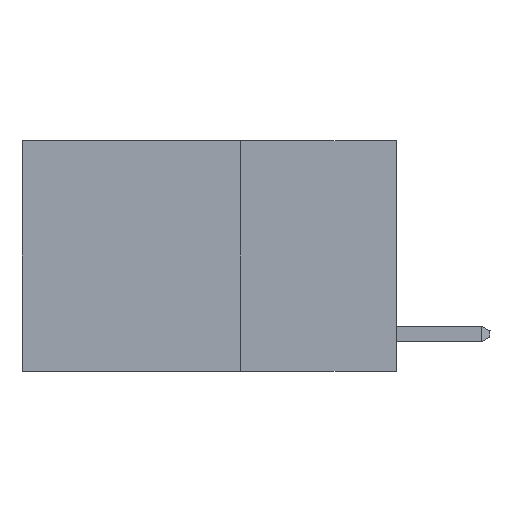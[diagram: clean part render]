
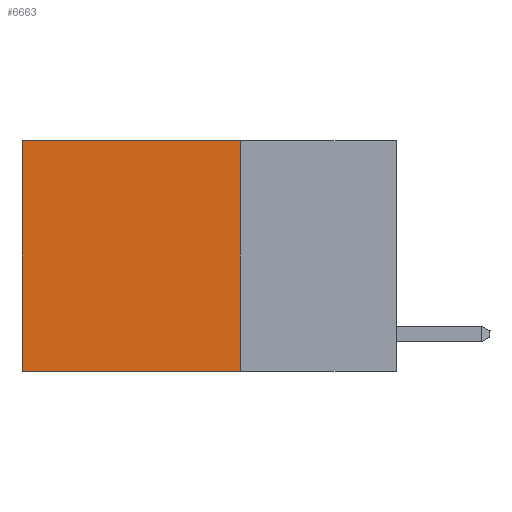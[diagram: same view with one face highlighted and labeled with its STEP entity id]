
A CAD part, left-side view. The second image highlights one B-rep face of the part: STEP entity #6663.
In plain terms, the highlighted planar face has unit normal (-1, 0, 0).
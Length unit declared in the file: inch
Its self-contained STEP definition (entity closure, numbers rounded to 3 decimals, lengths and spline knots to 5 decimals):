
#4 = CARTESIAN_POINT ( 'NONE',  ( 0.2625, 0.6, -0.37 ) ) ;
#720 = VECTOR ( 'NONE', #11246, 39.37008 ) ;
#1445 = LINE ( 'NONE', #13525, #2460 ) ;
#1889 = ORIENTED_EDGE ( 'NONE', *, *, #14683, .F. ) ;
#2210 = VERTEX_POINT ( 'NONE', #4 ) ;
#2460 = VECTOR ( 'NONE', #14860, 39.37008 ) ;
#6091 = DIRECTION ( 'NONE',  ( 1., 0., 0. ) ) ;
#6094 = VERTEX_POINT ( 'NONE', #7004 ) ;
#6663 = ADVANCED_FACE ( 'NONE', ( #11835 ), #9126, .F. ) ;
#6929 = LINE ( 'NONE', #12760, #720 ) ;
#7004 = CARTESIAN_POINT ( 'NONE',  ( 0.2625, 0.6, 0. ) ) ;
#7525 = CARTESIAN_POINT ( 'NONE',  ( 0.2625, 0.25, 0. ) ) ;
#7706 = LINE ( 'NONE', #15870, #15018 ) ;
#8579 = CARTESIAN_POINT ( 'NONE',  ( 0.2625, 0.25, 0. ) ) ;
#9126 = PLANE ( 'NONE',  #16337 ) ;
#9856 = ORIENTED_EDGE ( 'NONE', *, *, #15340, .T. ) ;
#10721 = VECTOR ( 'NONE', #12465, 39.37008 ) ;
#10777 = VERTEX_POINT ( 'NONE', #8579 ) ;
#11246 = DIRECTION ( 'NONE',  ( 0., 0., -1. ) ) ;
#11835 = FACE_OUTER_BOUND ( 'NONE', #15241, .T. ) ;
#11907 = EDGE_CURVE ( 'NONE', #10777, #6094, #16325, .T. ) ;
#12465 = DIRECTION ( 'NONE',  ( 0., 1., 0. ) ) ;
#12760 = CARTESIAN_POINT ( 'NONE',  ( 0.2625, 0.25, 0. ) ) ;
#12989 = DIRECTION ( 'NONE',  ( 0., 0., -1. ) ) ;
#13169 = DIRECTION ( 'NONE',  ( 0., 1., 0. ) ) ;
#13395 = ORIENTED_EDGE ( 'NONE', *, *, #11907, .T. ) ;
#13525 = CARTESIAN_POINT ( 'NONE',  ( 0.2625, 0.6, 0. ) ) ;
#13528 = EDGE_CURVE ( 'NONE', #15364, #2210, #7706, .T. ) ;
#14683 = EDGE_CURVE ( 'NONE', #10777, #15364, #6929, .T. ) ;
#14860 = DIRECTION ( 'NONE',  ( 0., 0., -1. ) ) ;
#15018 = VECTOR ( 'NONE', #13169, 39.37008 ) ;
#15241 = EDGE_LOOP ( 'NONE', ( #9856, #16349, #1889, #13395 ) ) ;
#15340 = EDGE_CURVE ( 'NONE', #6094, #2210, #1445, .T. ) ;
#15364 = VERTEX_POINT ( 'NONE', #17404 ) ;
#15870 = CARTESIAN_POINT ( 'NONE',  ( 0.2625, 0.25, -0.37 ) ) ;
#16325 = LINE ( 'NONE', #16506, #10721 ) ;
#16337 = AXIS2_PLACEMENT_3D ( 'NONE', #7525, #6091, #12989 ) ;
#16349 = ORIENTED_EDGE ( 'NONE', *, *, #13528, .F. ) ;
#16506 = CARTESIAN_POINT ( 'NONE',  ( 0.2625, 0.25, 0. ) ) ;
#17404 = CARTESIAN_POINT ( 'NONE',  ( 0.2625, 0.25, -0.37 ) ) ;
